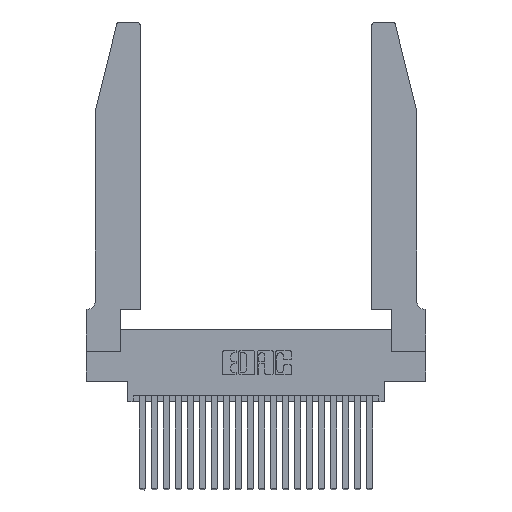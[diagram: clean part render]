
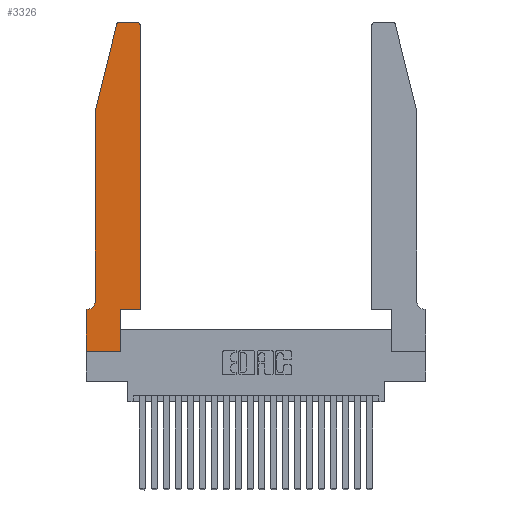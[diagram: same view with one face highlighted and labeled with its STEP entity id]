
A CAD part, top view. The second image highlights one B-rep face of the part: STEP entity #3326.
In plain terms, the highlighted planar face has unit normal (0, 0, 1).
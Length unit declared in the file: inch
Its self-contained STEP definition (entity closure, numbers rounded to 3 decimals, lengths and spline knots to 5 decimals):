
#18 = ORIENTED_EDGE ( 'NONE', *, *, #2637, .T. ) ;
#88 = CARTESIAN_POINT ( 'NONE',  ( 0., 0.35, 0.37 ) ) ;
#164 = EDGE_CURVE ( 'NONE', #6002, #19086, #21842, .T. ) ;
#281 = CARTESIAN_POINT ( 'NONE',  ( 0.4205, 2.72, 0.37 ) ) ;
#390 = LINE ( 'NONE', #20716, #19001 ) ;
#719 = CARTESIAN_POINT ( 'NONE',  ( 0.0055, 0.42, 0.37 ) ) ;
#728 = VERTEX_POINT ( 'NONE', #18556 ) ;
#888 = CARTESIAN_POINT ( 'NONE',  ( 0.0755, 2., 0.37 ) ) ;
#1240 = CARTESIAN_POINT ( 'NONE',  ( 0.2865, 0.35, 0.37 ) ) ;
#1319 = AXIS2_PLACEMENT_3D ( 'NONE', #719, #2773, #20577 ) ;
#1633 = EDGE_CURVE ( 'NONE', #20336, #18476, #21512, .T. ) ;
#2637 = EDGE_CURVE ( 'NONE', #21217, #728, #4539, .T. ) ;
#2711 = VECTOR ( 'NONE', #12688, 39.37008 ) ;
#2773 = DIRECTION ( 'NONE',  ( 0., 0., -1. ) ) ;
#2801 = CARTESIAN_POINT ( 'NONE',  ( 0.4505, 0.35, 0.37 ) ) ;
#2848 = DIRECTION ( 'NONE',  ( 0., 1., 0. ) ) ;
#2974 = CARTESIAN_POINT ( 'NONE',  ( 0.2865, 0.35, 0.37 ) ) ;
#3326 = ADVANCED_FACE ( 'NONE', ( #10709 ), #13195, .T. ) ;
#3345 = EDGE_CURVE ( 'NONE', #18476, #10295, #9564, .T. ) ;
#3350 = ORIENTED_EDGE ( 'NONE', *, *, #7186, .T. ) ;
#3361 = CARTESIAN_POINT ( 'NONE',  ( 0.4505, 0.35, 0.37 ) ) ;
#3907 = ORIENTED_EDGE ( 'NONE', *, *, #1633, .T. ) ;
#4098 = DIRECTION ( 'NONE',  ( 1., 0., 0. ) ) ;
#4311 = CARTESIAN_POINT ( 'NONE',  ( 0.284, 2.72, 0.37 ) ) ;
#4539 = LINE ( 'NONE', #21591, #14146 ) ;
#4558 = VERTEX_POINT ( 'NONE', #14708 ) ;
#4597 = CIRCLE ( 'NONE', #22692, 0.03 ) ;
#5254 = EDGE_CURVE ( 'NONE', #10295, #5386, #16293, .T. ) ;
#5386 = VERTEX_POINT ( 'NONE', #21971 ) ;
#6002 = VERTEX_POINT ( 'NONE', #12156 ) ;
#6053 = CARTESIAN_POINT ( 'NONE',  ( 0., 0.35, 0.37 ) ) ;
#6226 = VECTOR ( 'NONE', #13670, 39.37008 ) ;
#7186 = EDGE_CURVE ( 'NONE', #16133, #4558, #390, .T. ) ;
#7610 = CARTESIAN_POINT ( 'NONE',  ( 0.4205, 2.75, 0.37 ) ) ;
#7948 = DIRECTION ( 'NONE',  ( 0., 0., 1. ) ) ;
#8080 = VECTOR ( 'NONE', #15588, 39.37008 ) ;
#8151 = DIRECTION ( 'NONE',  ( 0., -1., 0. ) ) ;
#8334 = ORIENTED_EDGE ( 'NONE', *, *, #12033, .T. ) ;
#8384 = ORIENTED_EDGE ( 'NONE', *, *, #3345, .T. ) ;
#8408 = ORIENTED_EDGE ( 'NONE', *, *, #8428, .T. ) ;
#8422 = ORIENTED_EDGE ( 'NONE', *, *, #18925, .T. ) ;
#8428 = EDGE_CURVE ( 'NONE', #19086, #21217, #13308, .T. ) ;
#9564 = LINE ( 'NONE', #888, #6226 ) ;
#9758 = AXIS2_PLACEMENT_3D ( 'NONE', #4311, #7948, #13437 ) ;
#9761 = ORIENTED_EDGE ( 'NONE', *, *, #5254, .T. ) ;
#10229 = EDGE_LOOP ( 'NONE', ( #11745, #3907, #8384, #9761, #8334, #12722, #8408, #18, #19286, #8422, #3350, #15048 ) ) ;
#10295 = VERTEX_POINT ( 'NONE', #15315 ) ;
#10709 = FACE_OUTER_BOUND ( 'NONE', #10229, .T. ) ;
#10867 = DIRECTION ( 'NONE',  ( 1., 0., 0. ) ) ;
#10878 = CARTESIAN_POINT ( 'NONE',  ( 0.0755, 2., 0.37 ) ) ;
#11097 = CARTESIAN_POINT ( 'NONE',  ( 0.284, 2.75, 0.37 ) ) ;
#11745 = ORIENTED_EDGE ( 'NONE', *, *, #13875, .T. ) ;
#11767 = DIRECTION ( 'NONE',  ( 0., 0., 1. ) ) ;
#11907 = CARTESIAN_POINT ( 'NONE',  ( 0., 0., 0.37 ) ) ;
#12033 = EDGE_CURVE ( 'NONE', #5386, #6002, #13725, .T. ) ;
#12156 = CARTESIAN_POINT ( 'NONE',  ( 0.0055, 0.35, 0.37 ) ) ;
#12247 = VECTOR ( 'NONE', #19682, 39.37008 ) ;
#12605 = LINE ( 'NONE', #3361, #19312 ) ;
#12688 = DIRECTION ( 'NONE',  ( 0., -1., 0. ) ) ;
#12722 = ORIENTED_EDGE ( 'NONE', *, *, #164, .T. ) ;
#13151 = LINE ( 'NONE', #2974, #8080 ) ;
#13176 = EDGE_CURVE ( 'NONE', #728, #22719, #13151, .T. ) ;
#13195 = PLANE ( 'NONE',  #21576 ) ;
#13308 = LINE ( 'NONE', #11907, #21780 ) ;
#13437 = DIRECTION ( 'NONE',  ( 1., 0., 0. ) ) ;
#13670 = DIRECTION ( 'NONE',  ( -0.239, -0.971, 0. ) ) ;
#13725 = CIRCLE ( 'NONE', #1319, 0.07 ) ;
#13875 = EDGE_CURVE ( 'NONE', #19212, #20336, #14829, .T. ) ;
#14146 = VECTOR ( 'NONE', #10867, 39.37008 ) ;
#14704 = DIRECTION ( 'NONE',  ( -1., 0., 0. ) ) ;
#14708 = CARTESIAN_POINT ( 'NONE',  ( 0.4505, 2.72, 0.37 ) ) ;
#14829 = LINE ( 'NONE', #23228, #21578 ) ;
#15048 = ORIENTED_EDGE ( 'NONE', *, *, #15113, .T. ) ;
#15113 = EDGE_CURVE ( 'NONE', #4558, #19212, #4597, .T. ) ;
#15315 = CARTESIAN_POINT ( 'NONE',  ( 0.0755, 2., 0.37 ) ) ;
#15405 = DIRECTION ( 'NONE',  ( 1., 0., 0. ) ) ;
#15588 = DIRECTION ( 'NONE',  ( 0., 1., 0. ) ) ;
#16133 = VERTEX_POINT ( 'NONE', #2801 ) ;
#16293 = LINE ( 'NONE', #10878, #2711 ) ;
#16613 = CARTESIAN_POINT ( 'NONE',  ( 0., 0., 0.37 ) ) ;
#17685 = DIRECTION ( 'NONE',  ( 1., 0., 0. ) ) ;
#17879 = CARTESIAN_POINT ( 'NONE',  ( 0.0755, 0.35, 0.37 ) ) ;
#18172 = CARTESIAN_POINT ( 'NONE',  ( 0.25487, 2.72718, 0.37 ) ) ;
#18476 = VERTEX_POINT ( 'NONE', #18172 ) ;
#18556 = CARTESIAN_POINT ( 'NONE',  ( 0.2865, 0., 0.37 ) ) ;
#18925 = EDGE_CURVE ( 'NONE', #22719, #16133, #12605, .T. ) ;
#19001 = VECTOR ( 'NONE', #2848, 39.37008 ) ;
#19086 = VERTEX_POINT ( 'NONE', #88 ) ;
#19212 = VERTEX_POINT ( 'NONE', #7610 ) ;
#19286 = ORIENTED_EDGE ( 'NONE', *, *, #13176, .T. ) ;
#19312 = VECTOR ( 'NONE', #17685, 39.37008 ) ;
#19682 = DIRECTION ( 'NONE',  ( -1., 0., 0. ) ) ;
#19837 = DIRECTION ( 'NONE',  ( 0., 0., 1. ) ) ;
#20336 = VERTEX_POINT ( 'NONE', #11097 ) ;
#20577 = DIRECTION ( 'NONE',  ( -1., 0., 0. ) ) ;
#20716 = CARTESIAN_POINT ( 'NONE',  ( 0.4505, 0.35, 0.37 ) ) ;
#21217 = VERTEX_POINT ( 'NONE', #16613 ) ;
#21512 = CIRCLE ( 'NONE', #9758, 0.03 ) ;
#21576 = AXIS2_PLACEMENT_3D ( 'NONE', #6053, #11767, #15405 ) ;
#21578 = VECTOR ( 'NONE', #14704, 39.37008 ) ;
#21591 = CARTESIAN_POINT ( 'NONE',  ( 0., 0., 0.37 ) ) ;
#21780 = VECTOR ( 'NONE', #8151, 39.37008 ) ;
#21842 = LINE ( 'NONE', #17879, #12247 ) ;
#21971 = CARTESIAN_POINT ( 'NONE',  ( 0.0755, 0.42, 0.37 ) ) ;
#22692 = AXIS2_PLACEMENT_3D ( 'NONE', #281, #19837, #4098 ) ;
#22719 = VERTEX_POINT ( 'NONE', #1240 ) ;
#23228 = CARTESIAN_POINT ( 'NONE',  ( 0.2605, 2.75, 0.37 ) ) ;
